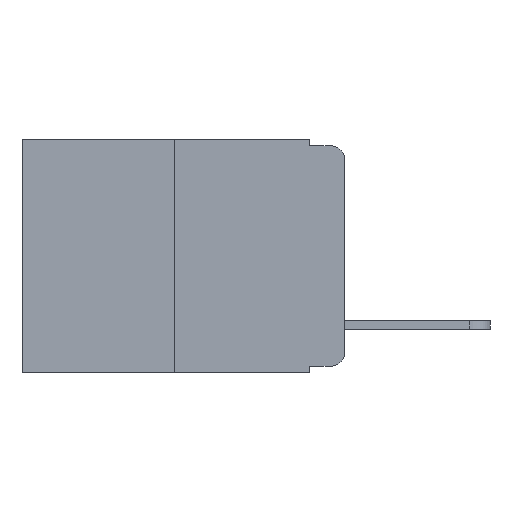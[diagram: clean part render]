
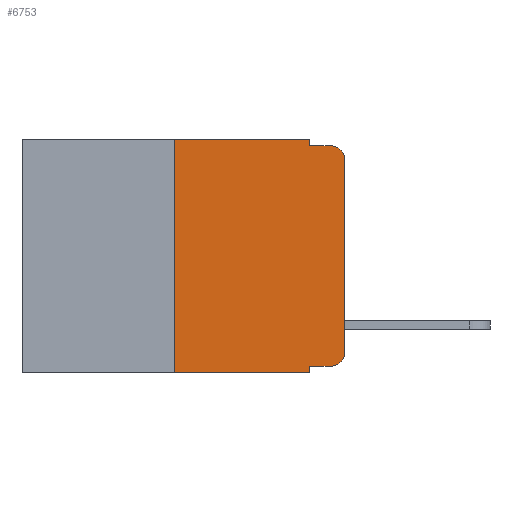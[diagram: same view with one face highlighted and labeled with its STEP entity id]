
A CAD part, left-side view. The second image highlights one B-rep face of the part: STEP entity #6753.
In plain terms, the highlighted planar face has unit normal (-1, 0, 0).
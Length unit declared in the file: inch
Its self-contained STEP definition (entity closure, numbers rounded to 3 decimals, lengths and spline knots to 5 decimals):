
#23 = ORIENTED_EDGE ( 'NONE', *, *, #14079, .T. ) ;
#34 = LINE ( 'NONE', #4862, #12431 ) ;
#356 = LINE ( 'NONE', #1952, #2286 ) ;
#396 = DIRECTION ( 'NONE',  ( 0., -1., 0. ) ) ;
#601 = EDGE_CURVE ( 'NONE', #10180, #10357, #356, .T. ) ;
#648 = EDGE_CURVE ( 'NONE', #1627, #10180, #6653, .T. ) ;
#970 = EDGE_CURVE ( 'NONE', #4635, #1627, #11621, .T. ) ;
#1600 = CARTESIAN_POINT ( 'NONE',  ( 0., 0.25, 0. ) ) ;
#1627 = VERTEX_POINT ( 'NONE', #1600 ) ;
#1731 = CARTESIAN_POINT ( 'NONE',  ( 0., 0.02, -0.03 ) ) ;
#1932 = DIRECTION ( 'NONE',  ( 1., 0., 0. ) ) ;
#1952 = CARTESIAN_POINT ( 'NONE',  ( 0., 0.051, 0. ) ) ;
#2042 = CARTESIAN_POINT ( 'NONE',  ( 0., 0.051, -0.01 ) ) ;
#2173 = ORIENTED_EDGE ( 'NONE', *, *, #8325, .T. ) ;
#2286 = VECTOR ( 'NONE', #6343, 39.37008 ) ;
#2460 = DIRECTION ( 'NONE',  ( 0., 0., -1. ) ) ;
#2893 = VECTOR ( 'NONE', #2460, 39.37008 ) ;
#3337 = VECTOR ( 'NONE', #8586, 39.37008 ) ;
#3417 = CARTESIAN_POINT ( 'NONE',  ( 0., 0., -0.03 ) ) ;
#3505 = DIRECTION ( 'NONE',  ( 0., 0., 1. ) ) ;
#3590 = ORIENTED_EDGE ( 'NONE', *, *, #14280, .F. ) ;
#3700 = EDGE_CURVE ( 'NONE', #10221, #8263, #7787, .T. ) ;
#3758 = AXIS2_PLACEMENT_3D ( 'NONE', #14387, #1932, #5487 ) ;
#3824 = EDGE_CURVE ( 'NONE', #10221, #9105, #34, .T. ) ;
#4188 = CARTESIAN_POINT ( 'NONE',  ( 0., 0.473, 0. ) ) ;
#4269 = VERTEX_POINT ( 'NONE', #12312 ) ;
#4323 = CARTESIAN_POINT ( 'NONE',  ( 0., 0., 0. ) ) ;
#4390 = DIRECTION ( 'NONE',  ( 0., -1., 0. ) ) ;
#4495 = LINE ( 'NONE', #4323, #12850 ) ;
#4520 = LINE ( 'NONE', #2042, #10134 ) ;
#4627 = EDGE_CURVE ( 'NONE', #4269, #6144, #4495, .T. ) ;
#4635 = VERTEX_POINT ( 'NONE', #5341 ) ;
#4862 = CARTESIAN_POINT ( 'NONE',  ( 0., 0.051, -0.333 ) ) ;
#5186 = CARTESIAN_POINT ( 'NONE',  ( 0., 0.051, -0.333 ) ) ;
#5312 = ORIENTED_EDGE ( 'NONE', *, *, #5472, .T. ) ;
#5341 = CARTESIAN_POINT ( 'NONE',  ( 0., 0.25, -0.343 ) ) ;
#5472 = EDGE_CURVE ( 'NONE', #9105, #4269, #10753, .T. ) ;
#5487 = DIRECTION ( 'NONE',  ( 0., 0., -1. ) ) ;
#5909 = VECTOR ( 'NONE', #13801, 39.37008 ) ;
#6144 = VERTEX_POINT ( 'NONE', #3417 ) ;
#6343 = DIRECTION ( 'NONE',  ( 0., 0., -1. ) ) ;
#6653 = LINE ( 'NONE', #4188, #3337 ) ;
#6753 = ADVANCED_FACE ( 'NONE', ( #8451 ), #8767, .F. ) ;
#7323 = DIRECTION ( 'NONE',  ( -1., 0., 0. ) ) ;
#7339 = EDGE_LOOP ( 'NONE', ( #12125, #2173, #3590, #13524, #14231, #12796, #23, #11667, #8594, #5312 ) ) ;
#7787 = LINE ( 'NONE', #10263, #2893 ) ;
#8263 = VERTEX_POINT ( 'NONE', #11662 ) ;
#8325 = EDGE_CURVE ( 'NONE', #6144, #12832, #8661, .T. ) ;
#8451 = FACE_OUTER_BOUND ( 'NONE', #7339, .T. ) ;
#8510 = CARTESIAN_POINT ( 'NONE',  ( 0., 0.02, -0.01 ) ) ;
#8554 = CARTESIAN_POINT ( 'NONE',  ( 0., 0.051, -0.01 ) ) ;
#8586 = DIRECTION ( 'NONE',  ( 0., -1., 0. ) ) ;
#8594 = ORIENTED_EDGE ( 'NONE', *, *, #3824, .T. ) ;
#8636 = VECTOR ( 'NONE', #3505, 39.37008 ) ;
#8661 = CIRCLE ( 'NONE', #11819, 0.02 ) ;
#8767 = PLANE ( 'NONE',  #3758 ) ;
#8887 = LINE ( 'NONE', #13945, #5909 ) ;
#9105 = VERTEX_POINT ( 'NONE', #12836 ) ;
#9303 = CARTESIAN_POINT ( 'NONE',  ( 0., 0.051, 0. ) ) ;
#9369 = AXIS2_PLACEMENT_3D ( 'NONE', #14074, #7323, #13683 ) ;
#9650 = DIRECTION ( 'NONE',  ( -1., 0., 0. ) ) ;
#10134 = VECTOR ( 'NONE', #4390, 39.37008 ) ;
#10180 = VERTEX_POINT ( 'NONE', #9303 ) ;
#10221 = VERTEX_POINT ( 'NONE', #5186 ) ;
#10263 = CARTESIAN_POINT ( 'NONE',  ( 0., 0.051, 0. ) ) ;
#10357 = VERTEX_POINT ( 'NONE', #8554 ) ;
#10753 = CIRCLE ( 'NONE', #9369, 0.02 ) ;
#11284 = CARTESIAN_POINT ( 'NONE',  ( 0., 0.25, 0. ) ) ;
#11621 = LINE ( 'NONE', #11284, #8636 ) ;
#11662 = CARTESIAN_POINT ( 'NONE',  ( 0., 0.051, -0.343 ) ) ;
#11667 = ORIENTED_EDGE ( 'NONE', *, *, #3700, .F. ) ;
#11798 = DIRECTION ( 'NONE',  ( 0., 0., -1. ) ) ;
#11819 = AXIS2_PLACEMENT_3D ( 'NONE', #1731, #9650, #11798 ) ;
#12125 = ORIENTED_EDGE ( 'NONE', *, *, #4627, .T. ) ;
#12129 = DIRECTION ( 'NONE',  ( 0., 0., 1. ) ) ;
#12312 = CARTESIAN_POINT ( 'NONE',  ( 0., 0., -0.313 ) ) ;
#12431 = VECTOR ( 'NONE', #396, 39.37008 ) ;
#12796 = ORIENTED_EDGE ( 'NONE', *, *, #970, .F. ) ;
#12832 = VERTEX_POINT ( 'NONE', #8510 ) ;
#12836 = CARTESIAN_POINT ( 'NONE',  ( 0., 0.02, -0.333 ) ) ;
#12850 = VECTOR ( 'NONE', #12129, 39.37008 ) ;
#13524 = ORIENTED_EDGE ( 'NONE', *, *, #601, .F. ) ;
#13683 = DIRECTION ( 'NONE',  ( 0., 0., -1. ) ) ;
#13801 = DIRECTION ( 'NONE',  ( 0., -1., 0. ) ) ;
#13945 = CARTESIAN_POINT ( 'NONE',  ( 0., 0.473, -0.343 ) ) ;
#14074 = CARTESIAN_POINT ( 'NONE',  ( 0., 0.02, -0.313 ) ) ;
#14079 = EDGE_CURVE ( 'NONE', #4635, #8263, #8887, .T. ) ;
#14231 = ORIENTED_EDGE ( 'NONE', *, *, #648, .F. ) ;
#14280 = EDGE_CURVE ( 'NONE', #10357, #12832, #4520, .T. ) ;
#14387 = CARTESIAN_POINT ( 'NONE',  ( 0., 0.473, 0. ) ) ;
